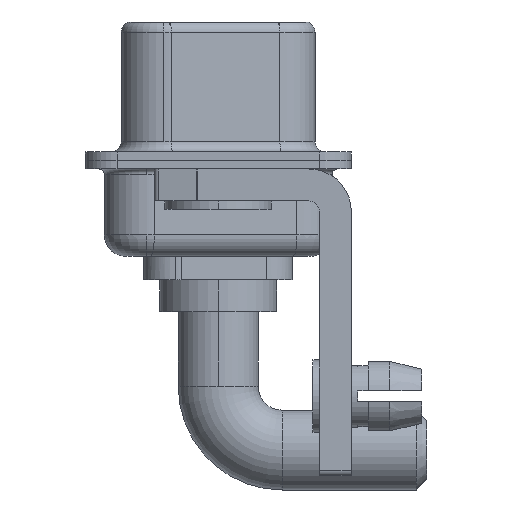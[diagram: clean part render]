
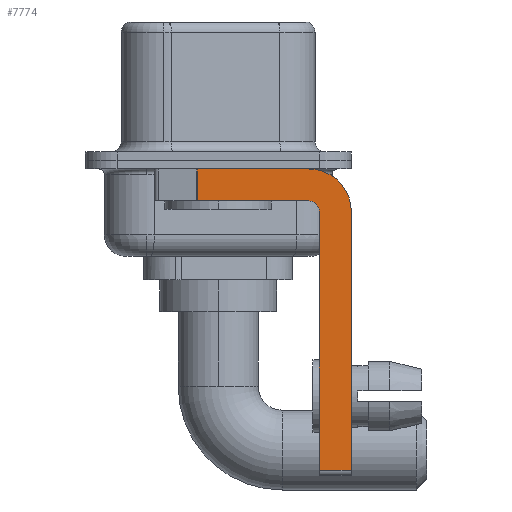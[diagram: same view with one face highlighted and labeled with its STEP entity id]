
A CAD part, left-side view. The second image highlights one B-rep face of the part: STEP entity #7774.
In plain terms, the highlighted planar face has unit normal (-1, 0, 0).
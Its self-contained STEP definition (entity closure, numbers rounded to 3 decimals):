
#42 = VECTOR ( 'NONE', #14887, 1000. ) ;
#158 = DIRECTION ( 'NONE',  ( 0., 0., -1. ) ) ;
#429 = CARTESIAN_POINT ( 'NONE',  ( -2.9, -4.25, -1.9 ) ) ;
#441 = ORIENTED_EDGE ( 'NONE', *, *, #482, .T. ) ;
#482 = EDGE_CURVE ( 'NONE', #15644, #13498, #10579, .T. ) ;
#909 = CARTESIAN_POINT ( 'NONE',  ( -2.9, -6.25, -14.55 ) ) ;
#1199 = AXIS2_PLACEMENT_3D ( 'NONE', #18368, #2938, #16973 ) ;
#1546 = VERTEX_POINT ( 'NONE', #15469 ) ;
#1894 = VECTOR ( 'NONE', #2348, 1000. ) ;
#2000 = EDGE_CURVE ( 'NONE', #2347, #15831, #3937, .T. ) ;
#2074 = LINE ( 'NONE', #16475, #1894 ) ;
#2347 = VERTEX_POINT ( 'NONE', #14960 ) ;
#2348 = DIRECTION ( 'NONE',  ( 0., 0., 1. ) ) ;
#2383 = AXIS2_PLACEMENT_3D ( 'NONE', #15961, #8590, #2782 ) ;
#2599 = ORIENTED_EDGE ( 'NONE', *, *, #13930, .F. ) ;
#2782 = DIRECTION ( 'NONE',  ( 0., 0., -1. ) ) ;
#2894 = CARTESIAN_POINT ( 'NONE',  ( -2.9, -4.25, -0.4 ) ) ;
#2938 = DIRECTION ( 'NONE',  ( -1., 0., 0. ) ) ;
#2958 = LINE ( 'NONE', #17448, #9004 ) ;
#3113 = ORIENTED_EDGE ( 'NONE', *, *, #11423, .F. ) ;
#3474 = CARTESIAN_POINT ( 'NONE',  ( -2.9, -4.25, -14.55 ) ) ;
#3937 = LINE ( 'NONE', #5438, #8532 ) ;
#4005 = VERTEX_POINT ( 'NONE', #14295 ) ;
#4176 = ORIENTED_EDGE ( 'NONE', *, *, #14094, .F. ) ;
#4179 = CARTESIAN_POINT ( 'NONE',  ( -2.9, -4.25, -2.4 ) ) ;
#5237 = ORIENTED_EDGE ( 'NONE', *, *, #18294, .F. ) ;
#5438 = CARTESIAN_POINT ( 'NONE',  ( -2.9, 0.978, -1.9 ) ) ;
#5489 = DIRECTION ( 'NONE',  ( 0., -1., 0. ) ) ;
#5773 = DIRECTION ( 'NONE',  ( 1., 0., 0. ) ) ;
#5811 = AXIS2_PLACEMENT_3D ( 'NONE', #4179, #5773, #14009 ) ;
#6927 = DIRECTION ( 'NONE',  ( 0., 0., -1. ) ) ;
#6978 = CARTESIAN_POINT ( 'NONE',  ( -2.9, 3., -0.4 ) ) ;
#7418 = LINE ( 'NONE', #6978, #11161 ) ;
#7623 = DIRECTION ( 'NONE',  ( 0., 1., 0. ) ) ;
#7768 = CIRCLE ( 'NONE', #1199, 0.5 ) ;
#7774 = ADVANCED_FACE ( 'NONE', ( #10251 ), #9979, .F. ) ;
#8342 = EDGE_CURVE ( 'NONE', #16993, #1546, #7768, .T. ) ;
#8532 = VECTOR ( 'NONE', #6927, 1000. ) ;
#8590 = DIRECTION ( 'NONE',  ( 1., 0., 0. ) ) ;
#9004 = VECTOR ( 'NONE', #158, 1000. ) ;
#9314 = ORIENTED_EDGE ( 'NONE', *, *, #16276, .F. ) ;
#9813 = CARTESIAN_POINT ( 'NONE',  ( -2.9, 0.978, -1.9 ) ) ;
#9979 = PLANE ( 'NONE',  #2383 ) ;
#10251 = FACE_OUTER_BOUND ( 'NONE', #10877, .T. ) ;
#10579 = LINE ( 'NONE', #3474, #42 ) ;
#10877 = EDGE_LOOP ( 'NONE', ( #9314, #15264, #4176, #16553, #3113, #441, #2599, #5237 ) ) ;
#10931 = CARTESIAN_POINT ( 'NONE',  ( -2.9, -4.75, -14.55 ) ) ;
#11161 = VECTOR ( 'NONE', #5489, 1000. ) ;
#11423 = EDGE_CURVE ( 'NONE', #15644, #16993, #2074, .T. ) ;
#13498 = VERTEX_POINT ( 'NONE', #909 ) ;
#13930 = EDGE_CURVE ( 'NONE', #4005, #13498, #2958, .T. ) ;
#14009 = DIRECTION ( 'NONE',  ( 0., 0., -1. ) ) ;
#14094 = EDGE_CURVE ( 'NONE', #1546, #15831, #16506, .T. ) ;
#14295 = CARTESIAN_POINT ( 'NONE',  ( -2.9, -6.25, -2.4 ) ) ;
#14785 = CARTESIAN_POINT ( 'NONE',  ( -2.9, -4.75, -2.4 ) ) ;
#14887 = DIRECTION ( 'NONE',  ( 0., -1., 0. ) ) ;
#14960 = CARTESIAN_POINT ( 'NONE',  ( -2.9, 0.978, -0.4 ) ) ;
#15264 = ORIENTED_EDGE ( 'NONE', *, *, #2000, .T. ) ;
#15469 = CARTESIAN_POINT ( 'NONE',  ( -2.9, -4.25, -1.9 ) ) ;
#15644 = VERTEX_POINT ( 'NONE', #10931 ) ;
#15778 = VERTEX_POINT ( 'NONE', #2894 ) ;
#15831 = VERTEX_POINT ( 'NONE', #9813 ) ;
#15874 = VECTOR ( 'NONE', #7623, 1000. ) ;
#15961 = CARTESIAN_POINT ( 'NONE',  ( -2.9, -4.25, -2.4 ) ) ;
#16276 = EDGE_CURVE ( 'NONE', #2347, #15778, #7418, .T. ) ;
#16475 = CARTESIAN_POINT ( 'NONE',  ( -2.9, -4.75, -14.8 ) ) ;
#16506 = LINE ( 'NONE', #429, #15874 ) ;
#16553 = ORIENTED_EDGE ( 'NONE', *, *, #8342, .F. ) ;
#16973 = DIRECTION ( 'NONE',  ( 0., 0., 1. ) ) ;
#16993 = VERTEX_POINT ( 'NONE', #14785 ) ;
#17448 = CARTESIAN_POINT ( 'NONE',  ( -2.9, -6.25, -2.4 ) ) ;
#17451 = CIRCLE ( 'NONE', #5811, 2. ) ;
#18294 = EDGE_CURVE ( 'NONE', #15778, #4005, #17451, .T. ) ;
#18368 = CARTESIAN_POINT ( 'NONE',  ( -2.9, -4.25, -2.4 ) ) ;
